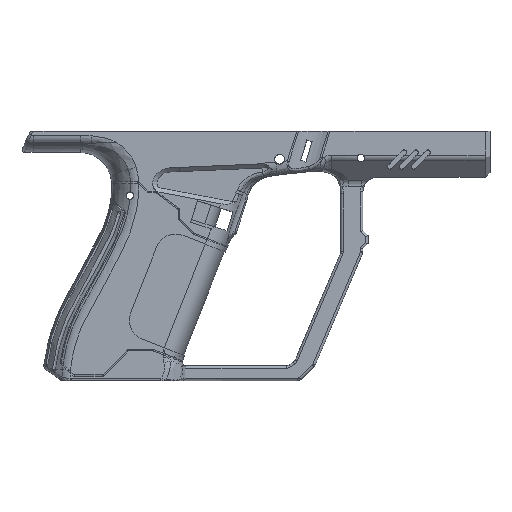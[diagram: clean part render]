
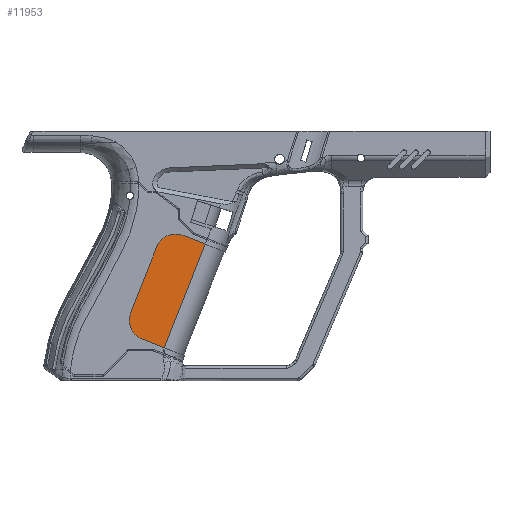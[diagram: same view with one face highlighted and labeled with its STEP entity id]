
A CAD part, top view. The second image highlights one B-rep face of the part: STEP entity #11953.
In plain terms, the highlighted planar face has unit normal (0, 0, 1).
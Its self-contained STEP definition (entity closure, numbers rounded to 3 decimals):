
#407=PLANE('',#12771);
#1739=FACE_OUTER_BOUND('',#2399,.T.);
#2399=EDGE_LOOP('',(#10503,#10504,#10505,#10506,#10507,#10508));
#3314=LINE('',#45872,#4118);
#3317=LINE('',#45878,#4121);
#3321=LINE('',#45915,#4125);
#3322=LINE('',#45919,#4126);
#4118=VECTOR('',#14958,1000.);
#4121=VECTOR('',#14963,1000.);
#4125=VECTOR('',#14973,1000.);
#4126=VECTOR('',#14980,1000.);
#4416=CIRCLE('',#12767,8.5);
#4417=CIRCLE('',#12770,8.5);
#5663=VERTEX_POINT('',#45713);
#5664=VERTEX_POINT('',#45871);
#5665=VERTEX_POINT('',#45875);
#5666=VERTEX_POINT('',#45877);
#5669=VERTEX_POINT('',#45909);
#5670=VERTEX_POINT('',#45913);
#7356=EDGE_CURVE('',#5664,#5663,#3314,.T.);
#7359=EDGE_CURVE('',#5666,#5665,#3317,.F.);
#7365=EDGE_CURVE('',#5665,#5669,#4416,.F.);
#7367=EDGE_CURVE('',#5669,#5670,#3321,.T.);
#7368=EDGE_CURVE('',#5670,#5664,#4417,.T.);
#7369=EDGE_CURVE('',#5663,#5666,#3322,.T.);
#10503=ORIENTED_EDGE('',*,*,#7369,.T.);
#10504=ORIENTED_EDGE('',*,*,#7359,.T.);
#10505=ORIENTED_EDGE('',*,*,#7365,.T.);
#10506=ORIENTED_EDGE('',*,*,#7367,.T.);
#10507=ORIENTED_EDGE('',*,*,#7368,.T.);
#10508=ORIENTED_EDGE('',*,*,#7356,.T.);
#11953=ADVANCED_FACE('',(#1739),#407,.F.);
#12767=AXIS2_PLACEMENT_3D('',#45911,#14968,#14969);
#12770=AXIS2_PLACEMENT_3D('',#45917,#14976,#14977);
#12771=AXIS2_PLACEMENT_3D('',#45918,#14978,#14979);
#14958=DIRECTION('',(0.93,-0.367,0.));
#14963=DIRECTION('',(0.93,-0.367,0.));
#14968=DIRECTION('center_axis',(0.,0.,
-1.));
#14969=DIRECTION('ref_axis',(-1.,0.,0.));
#14973=DIRECTION('',(-0.367,-0.93,0.));
#14976=DIRECTION('center_axis',(0.,0.,
1.));
#14977=DIRECTION('ref_axis',(-0.917,-0.399,0.));
#14978=DIRECTION('center_axis',(0.,0.,
-1.));
#14979=DIRECTION('ref_axis',(1.,0.,0.));
#14980=DIRECTION('',(0.367,0.93,0.));
#45713=CARTESIAN_POINT('',(265.216,-99.26,32.706));
#45871=CARTESIAN_POINT('',(255.966,-95.617,32.706));
#45872=CARTESIAN_POINT('',(255.966,-95.617,32.706));
#45875=CARTESIAN_POINT('',(273.082,-52.165,32.706));
#45877=CARTESIAN_POINT('',(282.332,-55.809,32.706));
#45878=CARTESIAN_POINT('',(282.132,-55.73,32.706));
#45909=CARTESIAN_POINT('',(262.058,-56.958,32.706));
#45911=CARTESIAN_POINT('Origin',(269.967,-60.073,32.706));
#45913=CARTESIAN_POINT('',(251.173,-84.593,32.706));
#45915=CARTESIAN_POINT('',(263.524,-53.236,32.706));
#45917=CARTESIAN_POINT('Origin',(259.081,-87.708,32.706));
#45918=CARTESIAN_POINT('Origin',(279.154,-63.291,32.706));
#45919=CARTESIAN_POINT('',(265.216,-99.26,32.706));
